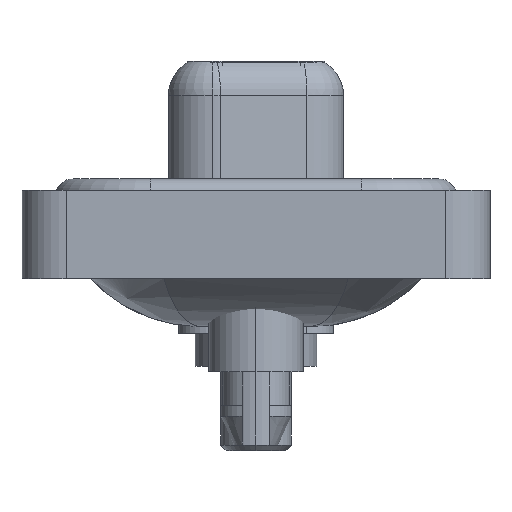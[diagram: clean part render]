
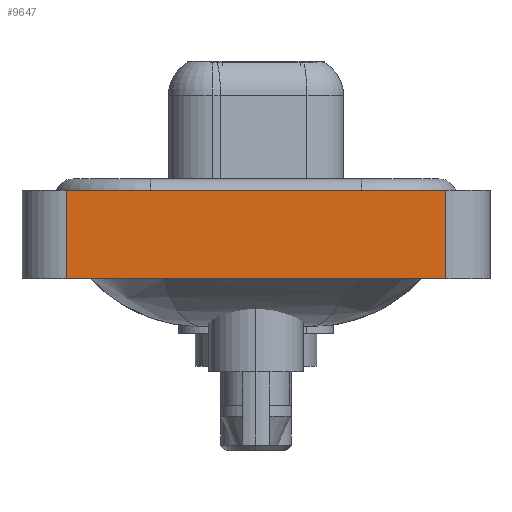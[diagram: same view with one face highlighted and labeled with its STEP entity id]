
A CAD part, left-side view. The second image highlights one B-rep face of the part: STEP entity #9647.
In plain terms, the highlighted planar face has unit normal (-1, 0, 0).
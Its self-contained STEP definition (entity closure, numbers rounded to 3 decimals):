
#405 = EDGE_CURVE ( 'NONE', #12110, #6110, #13537, .T. ) ;
#695 = CARTESIAN_POINT ( 'NONE',  ( -7.3, -8.55, 0.4 ) ) ;
#729 = CARTESIAN_POINT ( 'NONE',  ( -7.3, -8.55, -3.6 ) ) ;
#1140 = AXIS2_PLACEMENT_3D ( 'NONE', #11675, #1289, #6566 ) ;
#1289 = DIRECTION ( 'NONE',  ( -1., 0., 0. ) ) ;
#1682 = DIRECTION ( 'NONE',  ( 0., -1., 0. ) ) ;
#1687 = VECTOR ( 'NONE', #1682, 1000. ) ;
#1731 = CARTESIAN_POINT ( 'NONE',  ( -7.3, 8.55, 0.4 ) ) ;
#2040 = EDGE_CURVE ( 'NONE', #13438, #15703, #9424, .T. ) ;
#3527 = VECTOR ( 'NONE', #7099, 1000. ) ;
#3931 = PLANE ( 'NONE',  #1140 ) ;
#4296 = EDGE_CURVE ( 'NONE', #15703, #6110, #12166, .T. ) ;
#4533 = ORIENTED_EDGE ( 'NONE', *, *, #2040, .T. ) ;
#5950 = CARTESIAN_POINT ( 'NONE',  ( -7.3, -8.55, -3.6 ) ) ;
#6110 = VERTEX_POINT ( 'NONE', #695 ) ;
#6566 = DIRECTION ( 'NONE',  ( 0., 0., 1. ) ) ;
#6616 = ORIENTED_EDGE ( 'NONE', *, *, #11115, .F. ) ;
#7099 = DIRECTION ( 'NONE',  ( 0., -1., 0. ) ) ;
#9215 = FACE_OUTER_BOUND ( 'NONE', #12227, .T. ) ;
#9424 = LINE ( 'NONE', #10506, #1687 ) ;
#9564 = CARTESIAN_POINT ( 'NONE',  ( -7.3, 8.55, -3.6 ) ) ;
#9647 = ADVANCED_FACE ( 'NONE', ( #9215 ), #3931, .T. ) ;
#10186 = LINE ( 'NONE', #14252, #15815 ) ;
#10326 = ORIENTED_EDGE ( 'NONE', *, *, #4296, .T. ) ;
#10338 = VECTOR ( 'NONE', #10916, 1000. ) ;
#10506 = CARTESIAN_POINT ( 'NONE',  ( -7.3, -8.55, -3.6 ) ) ;
#10916 = DIRECTION ( 'NONE',  ( 0., 0., 1. ) ) ;
#11115 = EDGE_CURVE ( 'NONE', #13438, #12110, #10186, .T. ) ;
#11656 = ORIENTED_EDGE ( 'NONE', *, *, #405, .F. ) ;
#11675 = CARTESIAN_POINT ( 'NONE',  ( -7.3, -8.55, -3.6 ) ) ;
#12110 = VERTEX_POINT ( 'NONE', #1731 ) ;
#12166 = LINE ( 'NONE', #5950, #10338 ) ;
#12227 = EDGE_LOOP ( 'NONE', ( #10326, #11656, #6616, #4533 ) ) ;
#12948 = DIRECTION ( 'NONE',  ( 0., 0., 1. ) ) ;
#13374 = CARTESIAN_POINT ( 'NONE',  ( -7.3, -8.55, 0.4 ) ) ;
#13438 = VERTEX_POINT ( 'NONE', #9564 ) ;
#13537 = LINE ( 'NONE', #13374, #3527 ) ;
#14252 = CARTESIAN_POINT ( 'NONE',  ( -7.3, 8.55, -3.6 ) ) ;
#15703 = VERTEX_POINT ( 'NONE', #729 ) ;
#15815 = VECTOR ( 'NONE', #12948, 1000. ) ;
